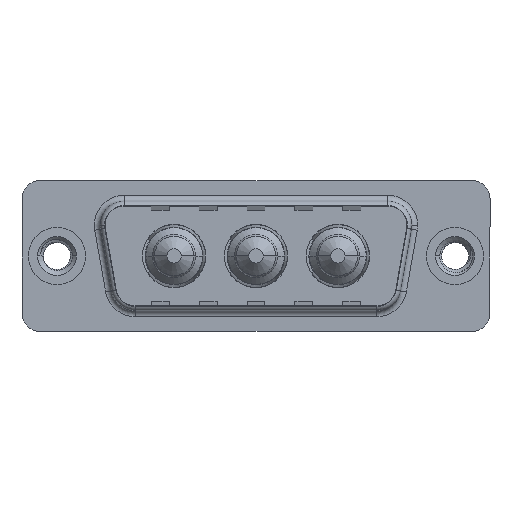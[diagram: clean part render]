
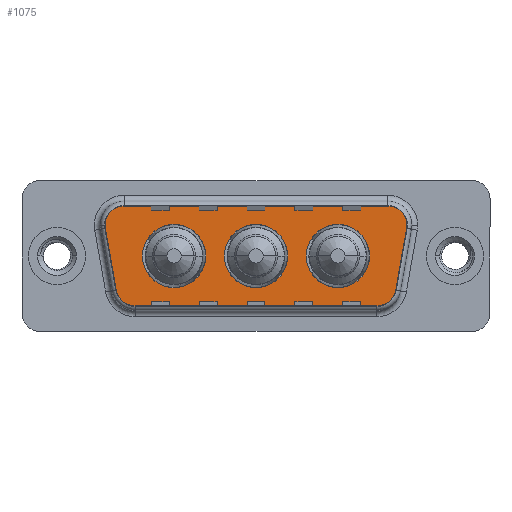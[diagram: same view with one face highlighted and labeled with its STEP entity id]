
A CAD part, top view. The second image highlights one B-rep face of the part: STEP entity #1075.
In plain terms, the highlighted planar face has unit normal (0, 0, 1).
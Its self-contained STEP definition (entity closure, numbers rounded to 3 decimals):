
#66 = EDGE_CURVE ( 'NONE', #13209, #4809, #7106, .T. ) ;
#68 = CARTESIAN_POINT ( 'NONE',  ( 27.889, 4.9, 0. ) ) ;
#103 = AXIS2_PLACEMENT_3D ( 'NONE', #9179, #3847, #14443 ) ;
#211 = CARTESIAN_POINT ( 'NONE',  ( 20.85, 0., 0. ) ) ;
#224 = CARTESIAN_POINT ( 'NONE',  ( 6.434, -4.9, 0. ) ) ;
#284 = EDGE_CURVE ( 'NONE', #14658, #2732, #11304, .T. ) ;
#390 = EDGE_CURVE ( 'NONE', #14608, #13356, #433, .T. ) ;
#417 = CARTESIAN_POINT ( 'NONE',  ( 6.434, -2.9, 0. ) ) ;
#433 = CIRCLE ( 'NONE', #9947, 2.65 ) ;
#435 = DIRECTION ( 'NONE',  ( -1., 0., 0. ) ) ;
#578 = EDGE_CURVE ( 'NONE', #10078, #2652, #1352, .T. ) ;
#591 = DIRECTION ( 'NONE',  ( -1., 0., 0. ) ) ;
#853 = EDGE_LOOP ( 'NONE', ( #10365, #13144 ) ) ;
#1075 = ADVANCED_FACE ( 'NONE', ( #6144, #9779, #9402, #12607 ), #12490, .T. ) ;
#1180 = ORIENTED_EDGE ( 'NONE', *, *, #5213, .T. ) ;
#1250 = ORIENTED_EDGE ( 'NONE', *, *, #9383, .T. ) ;
#1318 = CARTESIAN_POINT ( 'NONE',  ( 26.866, -2.9, 0. ) ) ;
#1350 = DIRECTION ( 'NONE',  ( 0., 0., 1. ) ) ;
#1352 = LINE ( 'NONE', #1645, #4656 ) ;
#1489 = AXIS2_PLACEMENT_3D ( 'NONE', #7170, #5555, #11831 ) ;
#1645 = CARTESIAN_POINT ( 'NONE',  ( 3.441, 2.553, 0. ) ) ;
#1770 = CARTESIAN_POINT ( 'NONE',  ( 16.65, 0., 0. ) ) ;
#2068 = EDGE_CURVE ( 'NONE', #4809, #13209, #5539, .T. ) ;
#2095 = DIRECTION ( 'NONE',  ( 0., 0., 1. ) ) ;
#2145 = ORIENTED_EDGE ( 'NONE', *, *, #4629, .T. ) ;
#2181 = ORIENTED_EDGE ( 'NONE', *, *, #10320, .F. ) ;
#2407 = DIRECTION ( 'NONE',  ( 0.174, -0.985, 0. ) ) ;
#2592 = CARTESIAN_POINT ( 'NONE',  ( 27.889, 2.9, 0. ) ) ;
#2652 = VERTEX_POINT ( 'NONE', #7871 ) ;
#2732 = VERTEX_POINT ( 'NONE', #211 ) ;
#2945 = CARTESIAN_POINT ( 'NONE',  ( 5.411, 4.9, 0. ) ) ;
#2973 = VECTOR ( 'NONE', #6965, 1000. ) ;
#2986 = EDGE_CURVE ( 'NONE', #2652, #9718, #11424, .T. ) ;
#3068 = ORIENTED_EDGE ( 'NONE', *, *, #8165, .T. ) ;
#3167 = CARTESIAN_POINT ( 'NONE',  ( 16.65, 0., 0. ) ) ;
#3340 = CARTESIAN_POINT ( 'NONE',  ( 3.441, 2.553, 0. ) ) ;
#3636 = ORIENTED_EDGE ( 'NONE', *, *, #4382, .T. ) ;
#3722 = VERTEX_POINT ( 'NONE', #13172 ) ;
#3847 = DIRECTION ( 'NONE',  ( 0., 0., 1. ) ) ;
#4149 = VECTOR ( 'NONE', #6431, 1000. ) ;
#4337 = VECTOR ( 'NONE', #7776, 1000. ) ;
#4357 = CIRCLE ( 'NONE', #11536, 2. ) ;
#4382 = EDGE_CURVE ( 'NONE', #6401, #10078, #13492, .T. ) ;
#4550 = AXIS2_PLACEMENT_3D ( 'NONE', #3167, #12710, #14947 ) ;
#4629 = EDGE_CURVE ( 'NONE', #5405, #5365, #4357, .T. ) ;
#4656 = VECTOR ( 'NONE', #2407, 1000. ) ;
#4667 = EDGE_LOOP ( 'NONE', ( #8157, #2181 ) ) ;
#4698 = DIRECTION ( 'NONE',  ( 1., 0., 0. ) ) ;
#4809 = VERTEX_POINT ( 'NONE', #10925 ) ;
#4912 = EDGE_CURVE ( 'NONE', #15289, #6401, #14213, .T. ) ;
#5127 = DIRECTION ( 'NONE',  ( -1., 0., 0. ) ) ;
#5213 = EDGE_CURVE ( 'NONE', #9718, #5405, #10833, .T. ) ;
#5365 = VERTEX_POINT ( 'NONE', #6049 ) ;
#5405 = VERTEX_POINT ( 'NONE', #13574 ) ;
#5539 = CIRCLE ( 'NONE', #9918, 2.65 ) ;
#5555 = DIRECTION ( 'NONE',  ( 0., 0., 1. ) ) ;
#5678 = CIRCLE ( 'NONE', #6437, 2.65 ) ;
#5848 = CARTESIAN_POINT ( 'NONE',  ( 7.15, 0., 0. ) ) ;
#6020 = EDGE_CURVE ( 'NONE', #3722, #15289, #15735, .T. ) ;
#6049 = CARTESIAN_POINT ( 'NONE',  ( 28.836, -3.247, 0. ) ) ;
#6144 = FACE_BOUND ( 'NONE', #853, .T. ) ;
#6148 = DIRECTION ( 'NONE',  ( 0., 0., 1. ) ) ;
#6196 = LINE ( 'NONE', #11820, #2973 ) ;
#6401 = VERTEX_POINT ( 'NONE', #15501 ) ;
#6431 = DIRECTION ( 'NONE',  ( -1., 0., 0. ) ) ;
#6437 = AXIS2_PLACEMENT_3D ( 'NONE', #13755, #6479, #14975 ) ;
#6479 = DIRECTION ( 'NONE',  ( 0., 0., 1. ) ) ;
#6668 = CARTESIAN_POINT ( 'NONE',  ( 12.45, 0., 0. ) ) ;
#6965 = DIRECTION ( 'NONE',  ( 0.174, 0.985, 0. ) ) ;
#7106 = CIRCLE ( 'NONE', #4550, 2.65 ) ;
#7170 = CARTESIAN_POINT ( 'NONE',  ( 26.866, -2.9, 0. ) ) ;
#7720 = DIRECTION ( 'NONE',  ( 0., 0., 1. ) ) ;
#7776 = DIRECTION ( 'NONE',  ( 1., 0., 0. ) ) ;
#7871 = CARTESIAN_POINT ( 'NONE',  ( 4.464, -3.247, 0. ) ) ;
#8157 = ORIENTED_EDGE ( 'NONE', *, *, #284, .F. ) ;
#8165 = EDGE_CURVE ( 'NONE', #5365, #10849, #6196, .T. ) ;
#8715 = AXIS2_PLACEMENT_3D ( 'NONE', #2592, #2095, #5127 ) ;
#9179 = CARTESIAN_POINT ( 'NONE',  ( 23.5, 0., 0. ) ) ;
#9363 = ORIENTED_EDGE ( 'NONE', *, *, #15480, .F. ) ;
#9383 = EDGE_CURVE ( 'NONE', #10849, #3722, #11591, .T. ) ;
#9402 = FACE_BOUND ( 'NONE', #10699, .T. ) ;
#9694 = CIRCLE ( 'NONE', #10980, 2.65 ) ;
#9718 = VERTEX_POINT ( 'NONE', #224 ) ;
#9779 = FACE_BOUND ( 'NONE', #4667, .T. ) ;
#9918 = AXIS2_PLACEMENT_3D ( 'NONE', #1770, #10905, #4698 ) ;
#9947 = AXIS2_PLACEMENT_3D ( 'NONE', #13911, #14959, #15509 ) ;
#10078 = VERTEX_POINT ( 'NONE', #3340 ) ;
#10320 = EDGE_CURVE ( 'NONE', #2732, #14658, #9694, .T. ) ;
#10365 = ORIENTED_EDGE ( 'NONE', *, *, #66, .F. ) ;
#10647 = AXIS2_PLACEMENT_3D ( 'NONE', #417, #1350, #591 ) ;
#10699 = EDGE_LOOP ( 'NONE', ( #15568, #9363 ) ) ;
#10833 = LINE ( 'NONE', #13440, #4337 ) ;
#10849 = VERTEX_POINT ( 'NONE', #10878 ) ;
#10878 = CARTESIAN_POINT ( 'NONE',  ( 29.859, 2.553, 0. ) ) ;
#10905 = DIRECTION ( 'NONE',  ( 0., 0., 1. ) ) ;
#10925 = CARTESIAN_POINT ( 'NONE',  ( 14., 0., 0. ) ) ;
#10963 = ORIENTED_EDGE ( 'NONE', *, *, #4912, .T. ) ;
#10976 = ORIENTED_EDGE ( 'NONE', *, *, #6020, .T. ) ;
#10980 = AXIS2_PLACEMENT_3D ( 'NONE', #13438, #6148, #14638 ) ;
#11166 = ORIENTED_EDGE ( 'NONE', *, *, #578, .T. ) ;
#11304 = CIRCLE ( 'NONE', #103, 2.65 ) ;
#11424 = CIRCLE ( 'NONE', #10647, 2. ) ;
#11536 = AXIS2_PLACEMENT_3D ( 'NONE', #1318, #13588, #14774 ) ;
#11591 = CIRCLE ( 'NONE', #15762, 2. ) ;
#11820 = CARTESIAN_POINT ( 'NONE',  ( 29.859, 2.553, 0. ) ) ;
#11831 = DIRECTION ( 'NONE',  ( 1., 0., 0. ) ) ;
#11954 = ORIENTED_EDGE ( 'NONE', *, *, #2986, .T. ) ;
#12120 = DIRECTION ( 'NONE',  ( 1., 0., 0. ) ) ;
#12303 = DIRECTION ( 'NONE',  ( 0., 0., 1. ) ) ;
#12490 = PLANE ( 'NONE',  #1489 ) ;
#12607 = FACE_OUTER_BOUND ( 'NONE', #15207, .T. ) ;
#12710 = DIRECTION ( 'NONE',  ( 0., 0., 1. ) ) ;
#13144 = ORIENTED_EDGE ( 'NONE', *, *, #2068, .F. ) ;
#13172 = CARTESIAN_POINT ( 'NONE',  ( 29.889, 2.9, 0. ) ) ;
#13209 = VERTEX_POINT ( 'NONE', #15394 ) ;
#13356 = VERTEX_POINT ( 'NONE', #5848 ) ;
#13438 = CARTESIAN_POINT ( 'NONE',  ( 23.5, 0., 0. ) ) ;
#13440 = CARTESIAN_POINT ( 'NONE',  ( 6.434, -4.9, 0. ) ) ;
#13470 = CARTESIAN_POINT ( 'NONE',  ( 5.411, 2.9, 0. ) ) ;
#13484 = AXIS2_PLACEMENT_3D ( 'NONE', #13470, #12303, #12120 ) ;
#13492 = CIRCLE ( 'NONE', #13484, 2. ) ;
#13574 = CARTESIAN_POINT ( 'NONE',  ( 26.866, -4.9, 0. ) ) ;
#13588 = DIRECTION ( 'NONE',  ( 0., 0., 1. ) ) ;
#13755 = CARTESIAN_POINT ( 'NONE',  ( 9.8, 0., 0. ) ) ;
#13911 = CARTESIAN_POINT ( 'NONE',  ( 9.8, 0., 0. ) ) ;
#14098 = CARTESIAN_POINT ( 'NONE',  ( 26.15, 0., 0. ) ) ;
#14213 = LINE ( 'NONE', #2945, #4149 ) ;
#14443 = DIRECTION ( 'NONE',  ( 1., 0., 0. ) ) ;
#14608 = VERTEX_POINT ( 'NONE', #6668 ) ;
#14638 = DIRECTION ( 'NONE',  ( 1., 0., 0. ) ) ;
#14658 = VERTEX_POINT ( 'NONE', #14098 ) ;
#14774 = DIRECTION ( 'NONE',  ( 1., 0., 0. ) ) ;
#14947 = DIRECTION ( 'NONE',  ( 1., 0., 0. ) ) ;
#14959 = DIRECTION ( 'NONE',  ( 0., 0., 1. ) ) ;
#14975 = DIRECTION ( 'NONE',  ( 1., 0., 0. ) ) ;
#15005 = CARTESIAN_POINT ( 'NONE',  ( 27.889, 2.9, 0. ) ) ;
#15207 = EDGE_LOOP ( 'NONE', ( #2145, #3068, #1250, #10976, #10963, #3636, #11166, #11954, #1180 ) ) ;
#15289 = VERTEX_POINT ( 'NONE', #68 ) ;
#15394 = CARTESIAN_POINT ( 'NONE',  ( 19.3, 0., 0. ) ) ;
#15480 = EDGE_CURVE ( 'NONE', #13356, #14608, #5678, .T. ) ;
#15501 = CARTESIAN_POINT ( 'NONE',  ( 5.411, 4.9, 0. ) ) ;
#15509 = DIRECTION ( 'NONE',  ( 1., 0., 0. ) ) ;
#15568 = ORIENTED_EDGE ( 'NONE', *, *, #390, .F. ) ;
#15735 = CIRCLE ( 'NONE', #8715, 2. ) ;
#15762 = AXIS2_PLACEMENT_3D ( 'NONE', #15005, #7720, #435 ) ;
